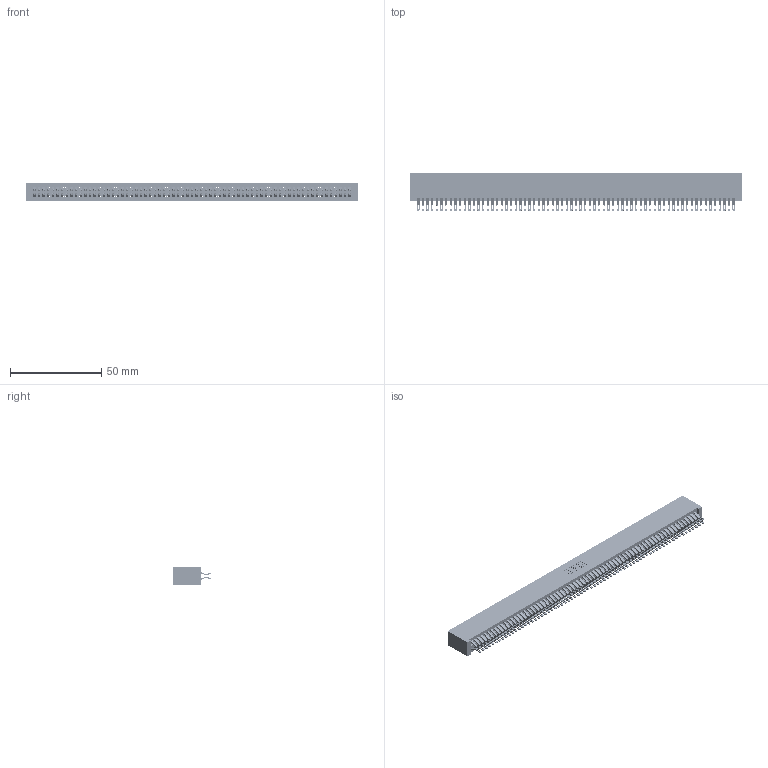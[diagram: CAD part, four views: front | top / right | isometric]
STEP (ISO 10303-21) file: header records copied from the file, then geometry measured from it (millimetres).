
FILE_DESCRIPTION (( 'STEP AP203' ), '1' );
FILE_NAME ('395-138-555-201.STEP', '2018-12-05T16:25:47', ( '' ), ( '' ), 'SwSTEP 2.0', 'SolidWorks 2016', '' );
FILE_SCHEMA (( 'CONFIG_CONTROL_DESIGN' ));
Length unit declared in the file: inch
Products named in the file (3): 345-292-001_555 Tail; 395-138-555-201; 345 Part_No Mounting Lugs
Assembly tree (139 placements, depth 2):
  395-138-555-201
    345 Part_No Mounting Lugs
    345-292-001_555 Tail  x138
Bounding box: 181.86 x 21.13 x 9.4 mm (x, y, z)
Volume: 18933.3 mm3; surface area: 30204.9 mm2
Topology: 139 solids, 139 shells, 7846 faces, 24743 edges, 16494 vertices
Faces by surface type: plane 4354, cylinder 3492
Entity records: 50553 total; most frequent: CARTESIAN_POINT 8482, ORIENTED_EDGE 8386, DIRECTION 7409, EDGE_CURVE 4193, LINE 3773, VECTOR 3773, VERTEX_POINT 2794, AXIS2_PLACEMENT_3D 1818
